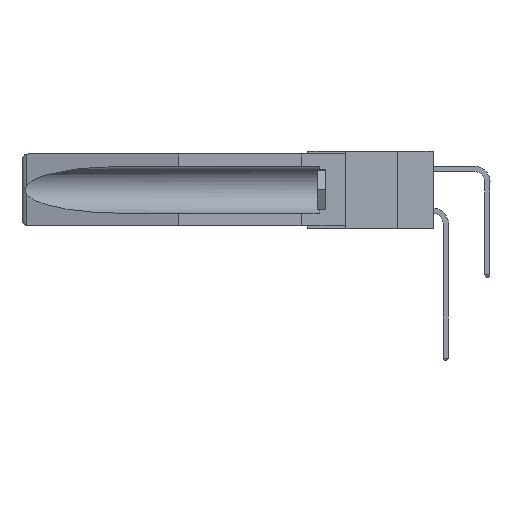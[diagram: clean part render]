
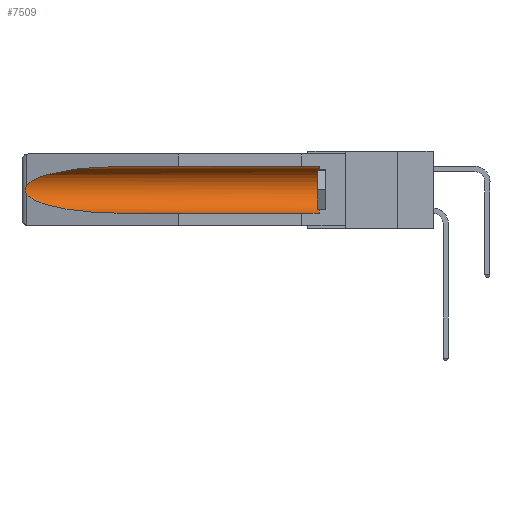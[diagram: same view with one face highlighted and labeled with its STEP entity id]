
A CAD part, left-side view. The second image highlights one B-rep face of the part: STEP entity #7509.
In plain terms, the highlighted cylindrical face has radius 2.857 mm (diameter 5.715 mm), a partial arc.
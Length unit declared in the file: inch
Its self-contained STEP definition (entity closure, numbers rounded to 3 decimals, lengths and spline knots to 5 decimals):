
#395 = LINE ( 'NONE', #9747, #7717 ) ;
#1047 = ORIENTED_EDGE ( 'NONE', *, *, #25855, .F. ) ;
#1143 = VERTEX_POINT ( 'NONE', #12661 ) ;
#1474 = CARTESIAN_POINT ( 'NONE',  ( 0.25451, 1.48313, -0.09465 ) ) ;
#1832 =( BOUNDED_CURVE ( )  B_SPLINE_CURVE ( 3, ( #4068, #16242, #1474, #24117 ),
 .UNSPECIFIED., .F., .T. ) 
 B_SPLINE_CURVE_WITH_KNOTS ( ( 4, 4 ),
 ( 4.71239, 6.08839 ),
 .UNSPECIFIED. ) 
 CURVE ( )  GEOMETRIC_REPRESENTATION_ITEM ( )  RATIONAL_B_SPLINE_CURVE ( ( 1., 0.848, 0.848, 1. ) ) 
 REPRESENTATION_ITEM ( '' )  );
#2247 = CARTESIAN_POINT ( 'NONE',  ( 0.155, 0.126, -0.1715 ) ) ;
#2792 = CARTESIAN_POINT ( 'NONE',  ( 0.155, -0.30754, -0.284 ) ) ;
#3581 = CARTESIAN_POINT ( 'NONE',  ( 0.155, 0.126, -0.284 ) ) ;
#4068 = CARTESIAN_POINT ( 'NONE',  ( 0.155, 1.07973, -0.059 ) ) ;
#4662 = ORIENTED_EDGE ( 'NONE', *, *, #26421, .T. ) ;
#4881 = CARTESIAN_POINT ( 'NONE',  ( 0.2675, 1.53308, -0.17534 ) ) ;
#4944 = VERTEX_POINT ( 'NONE', #12685 ) ;
#4997 = CARTESIAN_POINT ( 'NONE',  ( 0.26597, 1.52961, -0.15275 ) ) ;
#5007 = LINE ( 'NONE', #2792, #12696 ) ;
#5848 = CARTESIAN_POINT ( 'NONE',  ( 0.26537, 1.52718, -0.14972 ) ) ;
#5968 = CARTESIAN_POINT ( 'NONE',  ( 0.155, 1.07973, -0.284 ) ) ;
#7208 = CYLINDRICAL_SURFACE ( 'NONE', #22548, 0.1125 ) ;
#7254 = DIRECTION ( 'NONE',  ( 0., 1., 0. ) ) ;
#7480 = CARTESIAN_POINT ( 'NONE',  ( 0.26655, 1.53094, -0.18657 ) ) ;
#7509 = ADVANCED_FACE ( 'NONE', ( #17958 ), #7208, .F. ) ;
#7717 = VECTOR ( 'NONE', #7254, 39.37008 ) ;
#8390 = VERTEX_POINT ( 'NONE', #3581 ) ;
#8444 = CARTESIAN_POINT ( 'NONE',  ( 0.26537, 1.52718, -0.19328 ) ) ;
#8519 = CIRCLE ( 'NONE', #17505, 0.1125 ) ;
#8550 = ORIENTED_EDGE ( 'NONE', *, *, #28154, .T. ) ;
#9747 = CARTESIAN_POINT ( 'NONE',  ( 0.155, -0.30754, -0.059 ) ) ;
#10071 = CARTESIAN_POINT ( 'NONE',  ( 0.2673, 1.53269, -0.17917 ) ) ;
#10362 = EDGE_CURVE ( 'NONE', #21187, #21558, #1832, .T. ) ;
#10903 = B_SPLINE_CURVE_WITH_KNOTS ( 'NONE', 3,
 ( #29456, #4997, #29351, #24792, #17117, #4881, #10071, #7480, #27201, #29567 ),
 .UNSPECIFIED., .F., .F.,
 ( 4, 2, 2, 2, 4 ),
 ( 0., 0.00029, 0.00058, 0.00087, 0.00117 ),
 .UNSPECIFIED. ) ;
#11672 = ORIENTED_EDGE ( 'NONE', *, *, #31375, .T. ) ;
#12661 = CARTESIAN_POINT ( 'NONE',  ( 0.26537, 1.52718, -0.19328 ) ) ;
#12685 = CARTESIAN_POINT ( 'NONE',  ( 0.155, 0.126, -0.059 ) ) ;
#12696 = VECTOR ( 'NONE', #24929, 39.37008 ) ;
#14419 = EDGE_LOOP ( 'NONE', ( #26780, #4662, #11672, #1047, #8550, #29887 ) ) ;
#14558 = DIRECTION ( 'NONE',  ( 0., -1., 0. ) ) ;
#14573 = VERTEX_POINT ( 'NONE', #21266 ) ;
#16242 = CARTESIAN_POINT ( 'NONE',  ( 0.21114, 1.30732, -0.059 ) ) ;
#16479 = DIRECTION ( 'NONE',  ( 0., 1., 0. ) ) ;
#17117 = CARTESIAN_POINT ( 'NONE',  ( 0.2675, 1.53308, -0.16763 ) ) ;
#17505 = AXIS2_PLACEMENT_3D ( 'NONE', #2247, #14558, #19420 ) ;
#17958 = FACE_OUTER_BOUND ( 'NONE', #14419, .T. ) ;
#18208 = CARTESIAN_POINT ( 'NONE',  ( 0.155, 1.07973, -0.059 ) ) ;
#19079 = DIRECTION ( 'NONE',  ( 0., 0., 1. ) ) ;
#19420 = DIRECTION ( 'NONE',  ( 0., 0., 1. ) ) ;
#21187 = VERTEX_POINT ( 'NONE', #18208 ) ;
#21266 = CARTESIAN_POINT ( 'NONE',  ( 0.155, 1.07973, -0.284 ) ) ;
#21327 =( BOUNDED_CURVE ( )  B_SPLINE_CURVE ( 3, ( #8444, #22968, #25418, #5968 ),
 .UNSPECIFIED., .F., .F. ) 
 B_SPLINE_CURVE_WITH_KNOTS ( ( 4, 4 ),
 ( 0.1948, 1.5708 ),
 .UNSPECIFIED. ) 
 CURVE ( )  GEOMETRIC_REPRESENTATION_ITEM ( )  RATIONAL_B_SPLINE_CURVE ( ( 1., 0.848, 0.848, 1. ) ) 
 REPRESENTATION_ITEM ( '' )  );
#21558 = VERTEX_POINT ( 'NONE', #5848 ) ;
#22548 = AXIS2_PLACEMENT_3D ( 'NONE', #28718, #16479, #19079 ) ;
#22968 = CARTESIAN_POINT ( 'NONE',  ( 0.25451, 1.48313, -0.24835 ) ) ;
#24117 = CARTESIAN_POINT ( 'NONE',  ( 0.26537, 1.52718, -0.14972 ) ) ;
#24792 = CARTESIAN_POINT ( 'NONE',  ( 0.2673, 1.5327, -0.16383 ) ) ;
#24929 = DIRECTION ( 'NONE',  ( 0., 1., 0. ) ) ;
#25418 = CARTESIAN_POINT ( 'NONE',  ( 0.21114, 1.30732, -0.284 ) ) ;
#25855 = EDGE_CURVE ( 'NONE', #8390, #14573, #5007, .T. ) ;
#26421 = EDGE_CURVE ( 'NONE', #21558, #1143, #10903, .T. ) ;
#26780 = ORIENTED_EDGE ( 'NONE', *, *, #10362, .T. ) ;
#27201 = CARTESIAN_POINT ( 'NONE',  ( 0.26597, 1.5296, -0.19026 ) ) ;
#28154 = EDGE_CURVE ( 'NONE', #8390, #4944, #8519, .T. ) ;
#28718 = CARTESIAN_POINT ( 'NONE',  ( 0.155, -0.30754, -0.1715 ) ) ;
#28979 = EDGE_CURVE ( 'NONE', #4944, #21187, #395, .T. ) ;
#29351 = CARTESIAN_POINT ( 'NONE',  ( 0.26654, 1.53092, -0.15636 ) ) ;
#29456 = CARTESIAN_POINT ( 'NONE',  ( 0.26537, 1.52718, -0.14972 ) ) ;
#29567 = CARTESIAN_POINT ( 'NONE',  ( 0.26537, 1.52718, -0.19328 ) ) ;
#29887 = ORIENTED_EDGE ( 'NONE', *, *, #28979, .T. ) ;
#31375 = EDGE_CURVE ( 'NONE', #1143, #14573, #21327, .T. ) ;
